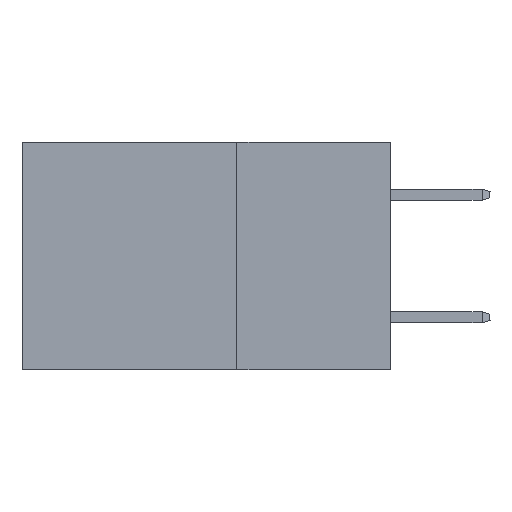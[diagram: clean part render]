
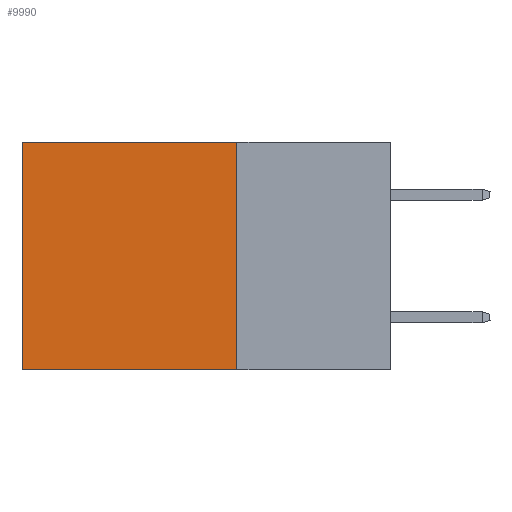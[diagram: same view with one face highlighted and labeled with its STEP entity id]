
A CAD part, left-side view. The second image highlights one B-rep face of the part: STEP entity #9990.
In plain terms, the highlighted planar face has unit normal (-1, 0, 0).
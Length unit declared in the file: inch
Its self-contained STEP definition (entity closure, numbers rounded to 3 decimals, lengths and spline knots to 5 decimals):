
#373 = DIRECTION ( 'NONE',  ( 0., 0., -1. ) ) ;
#853 = EDGE_CURVE ( 'NONE', #6225, #5189, #8249, .T. ) ;
#1067 = DIRECTION ( 'NONE',  ( 0., 0., -1. ) ) ;
#1128 = LINE ( 'NONE', #24868, #11125 ) ;
#1185 = AXIS2_PLACEMENT_3D ( 'NONE', #23647, #12298, #373 ) ;
#1461 = CARTESIAN_POINT ( 'NONE',  ( 0.2875, 0.6, 0. ) ) ;
#2872 = VECTOR ( 'NONE', #3370, 39.37008 ) ;
#3244 = CARTESIAN_POINT ( 'NONE',  ( 0.2875, 0.25, 0. ) ) ;
#3269 = CARTESIAN_POINT ( 'NONE',  ( 0.2875, 0.25, 0. ) ) ;
#3370 = DIRECTION ( 'NONE',  ( 0., 0., -1. ) ) ;
#5189 = VERTEX_POINT ( 'NONE', #7595 ) ;
#5497 = EDGE_CURVE ( 'NONE', #24320, #7836, #10815, .T. ) ;
#5691 = EDGE_CURVE ( 'NONE', #6225, #24320, #1128, .T. ) ;
#6225 = VERTEX_POINT ( 'NONE', #3244 ) ;
#7464 = LINE ( 'NONE', #13644, #18251 ) ;
#7595 = CARTESIAN_POINT ( 'NONE',  ( 0.2875, 0.25, -0.37 ) ) ;
#7836 = VERTEX_POINT ( 'NONE', #15986 ) ;
#8249 = LINE ( 'NONE', #3269, #2872 ) ;
#8394 = PLANE ( 'NONE',  #1185 ) ;
#8765 = ORIENTED_EDGE ( 'NONE', *, *, #5497, .T. ) ;
#9990 = ADVANCED_FACE ( 'NONE', ( #16328 ), #8394, .F. ) ;
#10526 = ORIENTED_EDGE ( 'NONE', *, *, #13959, .F. ) ;
#10815 = LINE ( 'NONE', #11019, #20935 ) ;
#11019 = CARTESIAN_POINT ( 'NONE',  ( 0.2875, 0.6, 0. ) ) ;
#11125 = VECTOR ( 'NONE', #15419, 39.37008 ) ;
#12298 = DIRECTION ( 'NONE',  ( 1., 0., 0. ) ) ;
#13595 = EDGE_LOOP ( 'NONE', ( #8765, #10526, #13660, #19938 ) ) ;
#13644 = CARTESIAN_POINT ( 'NONE',  ( 0.2875, 0.25, -0.37 ) ) ;
#13660 = ORIENTED_EDGE ( 'NONE', *, *, #853, .F. ) ;
#13959 = EDGE_CURVE ( 'NONE', #5189, #7836, #7464, .T. ) ;
#15419 = DIRECTION ( 'NONE',  ( 0., 1., 0. ) ) ;
#15986 = CARTESIAN_POINT ( 'NONE',  ( 0.2875, 0.6, -0.37 ) ) ;
#16328 = FACE_OUTER_BOUND ( 'NONE', #13595, .T. ) ;
#18251 = VECTOR ( 'NONE', #23163, 39.37008 ) ;
#19938 = ORIENTED_EDGE ( 'NONE', *, *, #5691, .T. ) ;
#20935 = VECTOR ( 'NONE', #1067, 39.37008 ) ;
#23163 = DIRECTION ( 'NONE',  ( 0., 1., 0. ) ) ;
#23647 = CARTESIAN_POINT ( 'NONE',  ( 0.2875, 0.25, 0. ) ) ;
#24320 = VERTEX_POINT ( 'NONE', #1461 ) ;
#24868 = CARTESIAN_POINT ( 'NONE',  ( 0.2875, 0.25, 0. ) ) ;
